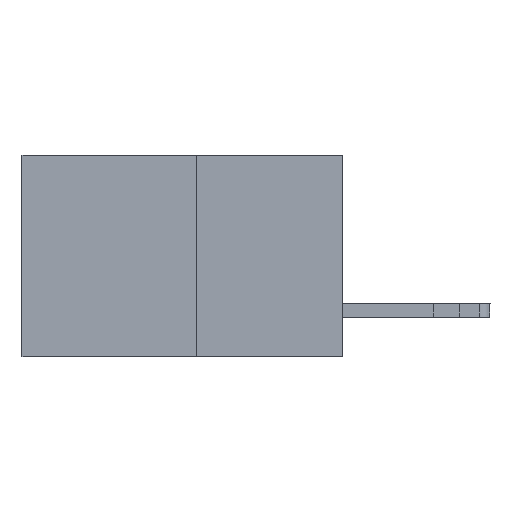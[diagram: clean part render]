
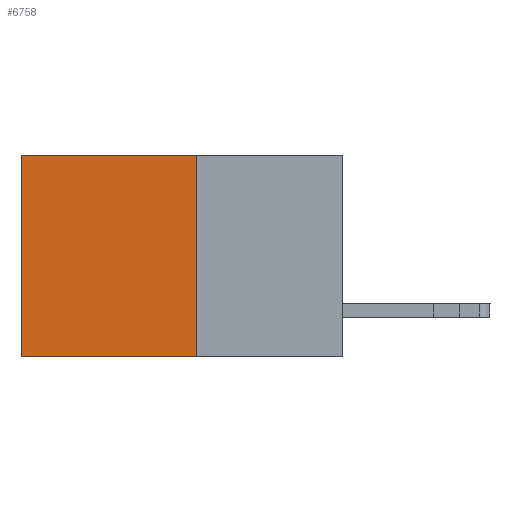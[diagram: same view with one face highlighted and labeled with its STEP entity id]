
A CAD part, left-side view. The second image highlights one B-rep face of the part: STEP entity #6758.
In plain terms, the highlighted planar face has unit normal (-1, 0, 0).
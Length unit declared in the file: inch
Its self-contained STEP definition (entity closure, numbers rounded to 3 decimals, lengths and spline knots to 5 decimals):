
#413 = LINE ( 'NONE', #16542, #14484 ) ;
#569 = VERTEX_POINT ( 'NONE', #14976 ) ;
#1316 = VERTEX_POINT ( 'NONE', #13433 ) ;
#2149 = DIRECTION ( 'NONE',  ( 0., 0., -1. ) ) ;
#2706 = VECTOR ( 'NONE', #12312, 39.37008 ) ;
#2851 = VECTOR ( 'NONE', #9822, 39.37008 ) ;
#3923 = LINE ( 'NONE', #5164, #7406 ) ;
#4022 = EDGE_CURVE ( 'NONE', #7125, #6476, #413, .T. ) ;
#4387 = PLANE ( 'NONE',  #6307 ) ;
#5164 = CARTESIAN_POINT ( 'NONE',  ( 0.277, 0.27, -0.37 ) ) ;
#6307 = AXIS2_PLACEMENT_3D ( 'NONE', #13570, #14875, #7020 ) ;
#6444 = CARTESIAN_POINT ( 'NONE',  ( 0.277, 0.59, 0. ) ) ;
#6463 = CARTESIAN_POINT ( 'NONE',  ( 0.277, 0.59, -0.37 ) ) ;
#6476 = VERTEX_POINT ( 'NONE', #6463 ) ;
#6758 = ADVANCED_FACE ( 'NONE', ( #15316 ), #4387, .F. ) ;
#6797 = ORIENTED_EDGE ( 'NONE', *, *, #12003, .F. ) ;
#7020 = DIRECTION ( 'NONE',  ( 0., 0., -1. ) ) ;
#7125 = VERTEX_POINT ( 'NONE', #6444 ) ;
#7158 = CARTESIAN_POINT ( 'NONE',  ( 0.277, 0.27, -0.37 ) ) ;
#7406 = VECTOR ( 'NONE', #15621, 39.37008 ) ;
#8071 = ORIENTED_EDGE ( 'NONE', *, *, #4022, .T. ) ;
#9822 = DIRECTION ( 'NONE',  ( 0., 1., 0. ) ) ;
#10286 = LINE ( 'NONE', #7158, #2851 ) ;
#10495 = EDGE_CURVE ( 'NONE', #569, #6476, #10286, .T. ) ;
#10980 = CARTESIAN_POINT ( 'NONE',  ( 0.277, 0.27, 0. ) ) ;
#11951 = EDGE_LOOP ( 'NONE', ( #8071, #13573, #6797, #14116 ) ) ;
#12003 = EDGE_CURVE ( 'NONE', #1316, #569, #3923, .T. ) ;
#12312 = DIRECTION ( 'NONE',  ( 0., 1., 0. ) ) ;
#12815 = LINE ( 'NONE', #10980, #2706 ) ;
#13433 = CARTESIAN_POINT ( 'NONE',  ( 0.277, 0.27, 0. ) ) ;
#13570 = CARTESIAN_POINT ( 'NONE',  ( 0.277, 0.27, -0.37 ) ) ;
#13573 = ORIENTED_EDGE ( 'NONE', *, *, #10495, .F. ) ;
#14116 = ORIENTED_EDGE ( 'NONE', *, *, #16826, .T. ) ;
#14484 = VECTOR ( 'NONE', #2149, 39.37008 ) ;
#14875 = DIRECTION ( 'NONE',  ( 1., 0., 0. ) ) ;
#14976 = CARTESIAN_POINT ( 'NONE',  ( 0.277, 0.27, -0.37 ) ) ;
#15316 = FACE_OUTER_BOUND ( 'NONE', #11951, .T. ) ;
#15621 = DIRECTION ( 'NONE',  ( 0., 0., -1. ) ) ;
#16542 = CARTESIAN_POINT ( 'NONE',  ( 0.277, 0.59, -0.37 ) ) ;
#16826 = EDGE_CURVE ( 'NONE', #1316, #7125, #12815, .T. ) ;
